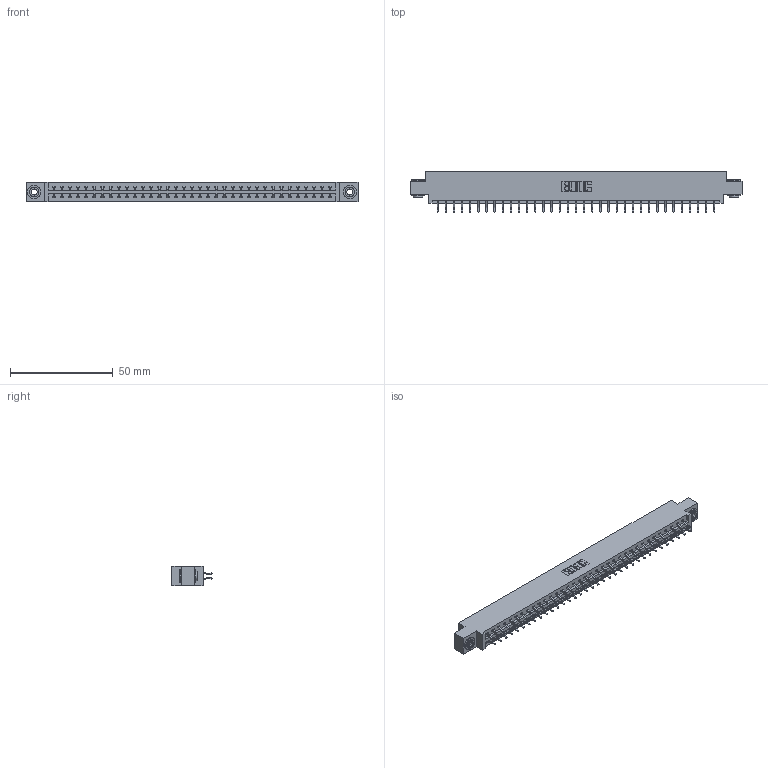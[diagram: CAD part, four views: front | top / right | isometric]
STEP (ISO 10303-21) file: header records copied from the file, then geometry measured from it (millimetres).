
FILE_DESCRIPTION (( 'STEP AP203' ), '1' );
FILE_NAME ('387-070-556-803.STEP', '2019-10-21T22:59:17', ( '' ), ( '' ), 'SwSTEP 2.0', 'SolidWorks 2016', '' );
FILE_SCHEMA (( 'CONFIG_CONTROL_DESIGN' ));
Length unit declared in the file: inch
Products named in the file (4): 387-070-556-803; 345-250-002_345-250-002-102; 337 Part_0.170 Offset - 0.156 Dia-TH; 345-292-001_556 Tail
Assembly tree (73 placements, depth 2):
  387-070-556-803
    337 Part_0.170 Offset - 0.156 Dia-TH
    345-292-001_556 Tail  x70
    345-250-002_345-250-002-102  x2
Bounding box: 161.7 x 19.57 x 9.4 mm (x, y, z)
Volume: 16846.8 mm3; surface area: 19235.7 mm2
Topology: 73 solids, 73 shells, 4356 faces, 12929 edges, 8522 vertices
Faces by surface type: plane 3024, cylinder 1324, cone 8
Entity records: 29044 total; most frequent: CARTESIAN_POINT 4889, ORIENTED_EDGE 4806, DIRECTION 4193, EDGE_CURVE 2403, VECTOR 2243, LINE 2243, VERTEX_POINT 1598, AXIS2_PLACEMENT_3D 975
